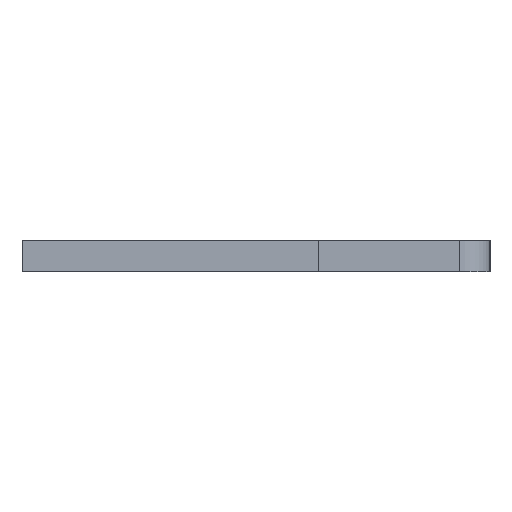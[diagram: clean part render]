
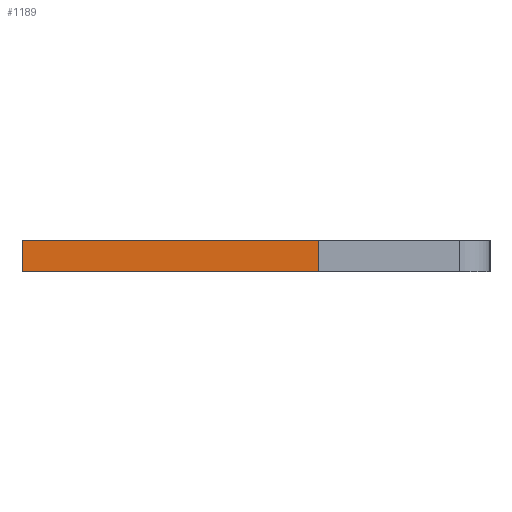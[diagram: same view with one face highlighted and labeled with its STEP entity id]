
A CAD part, left-side view. The second image highlights one B-rep face of the part: STEP entity #1189.
In plain terms, the highlighted face is planar.
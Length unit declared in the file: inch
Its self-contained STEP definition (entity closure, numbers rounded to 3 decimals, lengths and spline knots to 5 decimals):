
#17 = VECTOR ( 'NONE', #1497, 39.37008 ) ;
#74 = DIRECTION ( 'NONE',  ( -1., 0., 0. ) ) ;
#131 = CARTESIAN_POINT ( 'NONE',  ( 0.01, -0.04, -0.04 ) ) ;
#211 = LINE ( 'NONE', #1058, #1483 ) ;
#287 = CARTESIAN_POINT ( 'NONE',  ( 0.01, 0.15, -0.04 ) ) ;
#292 = VERTEX_POINT ( 'NONE', #1208 ) ;
#298 = CARTESIAN_POINT ( 'NONE',  ( 0.01, 0.15, -0.04 ) ) ;
#437 = ORIENTED_EDGE ( 'NONE', *, *, #1270, .T. ) ;
#508 = EDGE_CURVE ( 'NONE', #1225, #528, #211, .T. ) ;
#528 = VERTEX_POINT ( 'NONE', #2049 ) ;
#553 = ORIENTED_EDGE ( 'NONE', *, *, #751, .F. ) ;
#751 = EDGE_CURVE ( 'NONE', #1120, #528, #1808, .T. ) ;
#770 = DIRECTION ( 'NONE',  ( 0., 0., 1. ) ) ;
#807 = LINE ( 'NONE', #131, #1642 ) ;
#814 = FACE_OUTER_BOUND ( 'NONE', #1406, .T. ) ;
#954 = AXIS2_PLACEMENT_3D ( 'NONE', #298, #770, #1129 ) ;
#1058 = CARTESIAN_POINT ( 'NONE',  ( -0.01, 0.15, -0.04 ) ) ;
#1120 = VERTEX_POINT ( 'NONE', #287 ) ;
#1129 = DIRECTION ( 'NONE',  ( 1., 0., 0. ) ) ;
#1189 = ADVANCED_FACE ( 'NONE', ( #814 ), #1774, .F. ) ;
#1208 = CARTESIAN_POINT ( 'NONE',  ( 0.01, -0.04, -0.04 ) ) ;
#1225 = VERTEX_POINT ( 'NONE', #1452 ) ;
#1230 = DIRECTION ( 'NONE',  ( 0., 1., 0. ) ) ;
#1270 = EDGE_CURVE ( 'NONE', #292, #1225, #807, .T. ) ;
#1406 = EDGE_LOOP ( 'NONE', ( #1520, #553, #1505, #437 ) ) ;
#1452 = CARTESIAN_POINT ( 'NONE',  ( -0.01, -0.04, -0.04 ) ) ;
#1483 = VECTOR ( 'NONE', #1230, 39.37008 ) ;
#1497 = DIRECTION ( 'NONE',  ( 0., 1., 0. ) ) ;
#1505 = ORIENTED_EDGE ( 'NONE', *, *, #1614, .F. ) ;
#1520 = ORIENTED_EDGE ( 'NONE', *, *, #508, .T. ) ;
#1558 = LINE ( 'NONE', #1970, #17 ) ;
#1574 = CARTESIAN_POINT ( 'NONE',  ( 0.01, 0.15, -0.04 ) ) ;
#1610 = DIRECTION ( 'NONE',  ( -1., 0., 0. ) ) ;
#1614 = EDGE_CURVE ( 'NONE', #292, #1120, #1558, .T. ) ;
#1642 = VECTOR ( 'NONE', #1610, 39.37008 ) ;
#1702 = VECTOR ( 'NONE', #74, 39.37008 ) ;
#1774 = PLANE ( 'NONE',  #954 ) ;
#1808 = LINE ( 'NONE', #1574, #1702 ) ;
#1970 = CARTESIAN_POINT ( 'NONE',  ( 0.01, 0.15, -0.04 ) ) ;
#2049 = CARTESIAN_POINT ( 'NONE',  ( -0.01, 0.15, -0.04 ) ) ;
